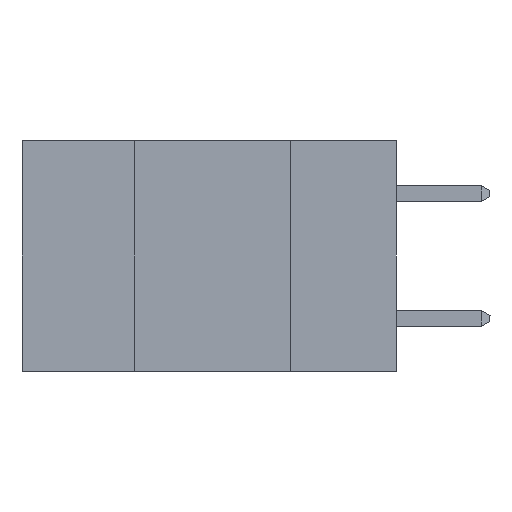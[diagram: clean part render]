
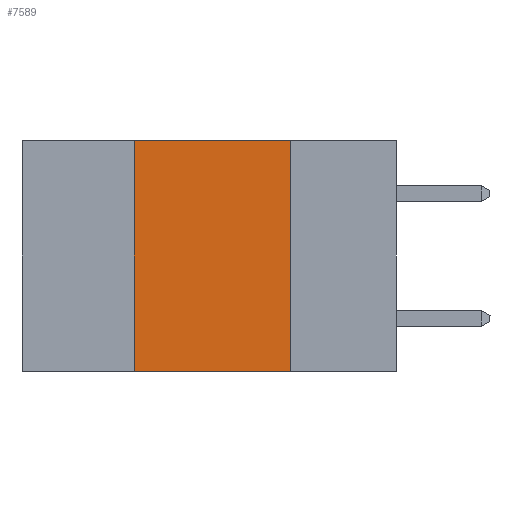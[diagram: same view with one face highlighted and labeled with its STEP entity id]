
A CAD part, left-side view. The second image highlights one B-rep face of the part: STEP entity #7589.
In plain terms, the highlighted planar face has unit normal (-1, 0, 0).
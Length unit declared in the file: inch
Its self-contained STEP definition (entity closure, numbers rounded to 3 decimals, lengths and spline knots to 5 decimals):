
#611 = EDGE_LOOP ( 'NONE', ( #10591, #4398, #1465, #15628 ) ) ;
#614 = EDGE_CURVE ( 'NONE', #1933, #4217, #15601, .T. ) ;
#735 = CARTESIAN_POINT ( 'NONE',  ( 0., 0.42, -0.37 ) ) ;
#1465 = ORIENTED_EDGE ( 'NONE', *, *, #11404, .F. ) ;
#1617 = CARTESIAN_POINT ( 'NONE',  ( 0., 0.6, -0.37 ) ) ;
#1918 = VECTOR ( 'NONE', #5016, 39.37008 ) ;
#1933 = VERTEX_POINT ( 'NONE', #4586 ) ;
#2086 = CARTESIAN_POINT ( 'NONE',  ( 0., 0.17, -0.37 ) ) ;
#2469 = DIRECTION ( 'NONE',  ( 0., 0., 1. ) ) ;
#2841 = VERTEX_POINT ( 'NONE', #735 ) ;
#3067 = EDGE_CURVE ( 'NONE', #2841, #4217, #8102, .T. ) ;
#3159 = CARTESIAN_POINT ( 'NONE',  ( 0., 0.17, -0.37 ) ) ;
#3211 = LINE ( 'NONE', #10921, #13028 ) ;
#4217 = VERTEX_POINT ( 'NONE', #3159 ) ;
#4398 = ORIENTED_EDGE ( 'NONE', *, *, #6622, .F. ) ;
#4586 = CARTESIAN_POINT ( 'NONE',  ( 0., 0.17, 0. ) ) ;
#5016 = DIRECTION ( 'NONE',  ( 0., -1., 0. ) ) ;
#5216 = VERTEX_POINT ( 'NONE', #14678 ) ;
#5431 = VECTOR ( 'NONE', #2469, 39.37008 ) ;
#5634 = DIRECTION ( 'NONE',  ( 0., 0., -1. ) ) ;
#6622 = EDGE_CURVE ( 'NONE', #5216, #1933, #3211, .T. ) ;
#7070 = DIRECTION ( 'NONE',  ( 1., 0., 0. ) ) ;
#7589 = ADVANCED_FACE ( 'NONE', ( #8821 ), #14403, .F. ) ;
#8102 = LINE ( 'NONE', #1617, #1918 ) ;
#8611 = CARTESIAN_POINT ( 'NONE',  ( 0., 0.42, -0.37 ) ) ;
#8821 = FACE_OUTER_BOUND ( 'NONE', #611, .T. ) ;
#10591 = ORIENTED_EDGE ( 'NONE', *, *, #614, .F. ) ;
#10921 = CARTESIAN_POINT ( 'NONE',  ( 0., 0.6, 0. ) ) ;
#11060 = DIRECTION ( 'NONE',  ( 0., -1., 0. ) ) ;
#11404 = EDGE_CURVE ( 'NONE', #2841, #5216, #15859, .T. ) ;
#13028 = VECTOR ( 'NONE', #11060, 39.37008 ) ;
#13214 = CARTESIAN_POINT ( 'NONE',  ( 0., 0.6, 0. ) ) ;
#14374 = AXIS2_PLACEMENT_3D ( 'NONE', #13214, #7070, #15563 ) ;
#14403 = PLANE ( 'NONE',  #14374 ) ;
#14509 = VECTOR ( 'NONE', #5634, 39.37008 ) ;
#14678 = CARTESIAN_POINT ( 'NONE',  ( 0., 0.42, 0. ) ) ;
#15563 = DIRECTION ( 'NONE',  ( 0., 0., -1. ) ) ;
#15601 = LINE ( 'NONE', #2086, #14509 ) ;
#15628 = ORIENTED_EDGE ( 'NONE', *, *, #3067, .T. ) ;
#15859 = LINE ( 'NONE', #8611, #5431 ) ;
